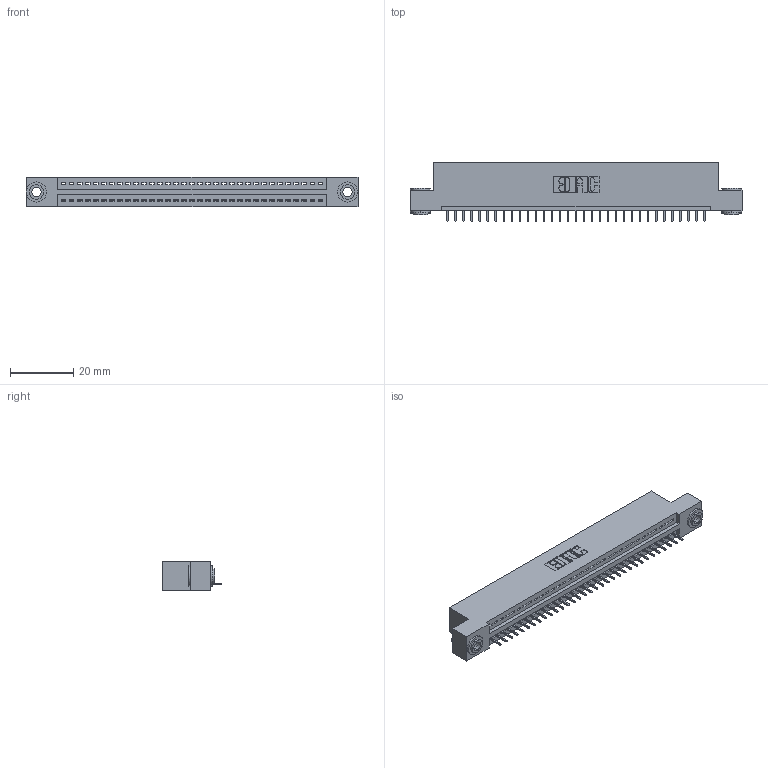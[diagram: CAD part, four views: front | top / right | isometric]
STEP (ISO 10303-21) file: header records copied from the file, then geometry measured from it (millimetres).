
FILE_DESCRIPTION (( 'STEP AP203' ), '1' );
FILE_NAME ('395-033-525-103.STEP', '2020-09-23T21:36:05', ( '' ), ( '' ), 'SwSTEP 2.0', 'SolidWorks 2020', '' );
FILE_SCHEMA (( 'CONFIG_CONTROL_DESIGN' ));
Length unit declared in the file: inch
Products named in the file (4): 345 Part_Flush Mounting Lugs - 0.156 Dia-TH; 345-250-002_345-250-002-102; 345-292-001_345-293-125; 395-033-525-103
Assembly tree (36 placements, depth 2):
  395-033-525-103
    345 Part_Flush Mounting Lugs - 0.156 Dia-TH
    345-292-001_345-293-125  x33
    345-250-002_345-250-002-102  x2
Bounding box: 105.03 x 18.72 x 9.4 mm (x, y, z)
Volume: 9786.7 mm3; surface area: 12648.5 mm2
Topology: 36 solids, 36 shells, 2210 faces, 6357 edges, 4102 vertices
Faces by surface type: plane 1608, cylinder 594, cone 8
Entity records: 26772 total; most frequent: CARTESIAN_POINT 4614, ORIENTED_EDGE 4574, DIRECTION 4075, EDGE_CURVE 2287, VECTOR 2003, LINE 2003, VERTEX_POINT 1518, AXIS2_PLACEMENT_3D 1036
